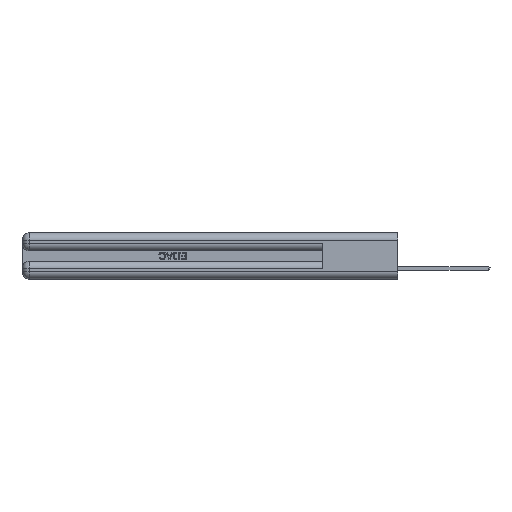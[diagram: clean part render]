
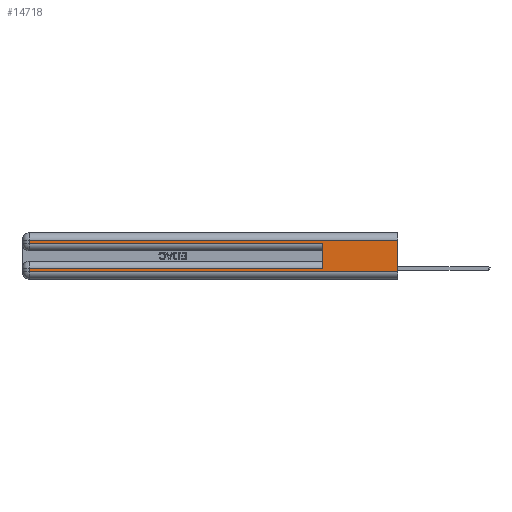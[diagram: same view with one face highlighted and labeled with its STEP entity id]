
A CAD part, left-side view. The second image highlights one B-rep face of the part: STEP entity #14718.
In plain terms, the highlighted planar face has unit normal (-1, 0, 0).
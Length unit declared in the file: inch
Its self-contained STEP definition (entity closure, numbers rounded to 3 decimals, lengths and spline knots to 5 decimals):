
#203 = CARTESIAN_POINT ( 'NONE',  ( 0., 2.94, 0.085 ) ) ;
#742 = DIRECTION ( 'NONE',  ( 0., 0., -1. ) ) ;
#860 = LINE ( 'NONE', #17339, #7563 ) ;
#980 = CARTESIAN_POINT ( 'NONE',  ( 0., 0., 0.06 ) ) ;
#1661 = LINE ( 'NONE', #35250, #13268 ) ;
#1668 = VECTOR ( 'NONE', #10809, 39.37008 ) ;
#3809 = VERTEX_POINT ( 'NONE', #30040 ) ;
#4321 = CARTESIAN_POINT ( 'NONE',  ( 0., 2.94, 0.37 ) ) ;
#5462 = VECTOR ( 'NONE', #8074, 39.37008 ) ;
#6271 = EDGE_CURVE ( 'NONE', #26611, #9084, #42999, .T. ) ;
#6389 = LINE ( 'NONE', #4321, #44031 ) ;
#6460 = CARTESIAN_POINT ( 'NONE',  ( 0., 2.94, 0.31 ) ) ;
#7563 = VECTOR ( 'NONE', #25642, 39.37008 ) ;
#8074 = DIRECTION ( 'NONE',  ( 0., 0., 1. ) ) ;
#8088 = DIRECTION ( 'NONE',  ( 0., 0., -1. ) ) ;
#8125 = FACE_OUTER_BOUND ( 'NONE', #28243, .T. ) ;
#9084 = VERTEX_POINT ( 'NONE', #203 ) ;
#9880 = ORIENTED_EDGE ( 'NONE', *, *, #37653, .T. ) ;
#10809 = DIRECTION ( 'NONE',  ( 0., 1., 0. ) ) ;
#11498 = CARTESIAN_POINT ( 'NONE',  ( 0., 0., 0.285 ) ) ;
#12879 = CARTESIAN_POINT ( 'NONE',  ( 0., 0.6, 0.285 ) ) ;
#13268 = VECTOR ( 'NONE', #23384, 39.37008 ) ;
#13643 = LINE ( 'NONE', #980, #31822 ) ;
#13735 = EDGE_CURVE ( 'NONE', #47105, #3809, #34945, .T. ) ;
#14718 = ADVANCED_FACE ( 'NONE', ( #8125 ), #19404, .F. ) ;
#14836 = VECTOR ( 'NONE', #22846, 39.37008 ) ;
#17339 = CARTESIAN_POINT ( 'NONE',  ( 0., 0., 0.31 ) ) ;
#18374 = EDGE_CURVE ( 'NONE', #9084, #39132, #1661, .T. ) ;
#19404 = PLANE ( 'NONE',  #20004 ) ;
#20004 = AXIS2_PLACEMENT_3D ( 'NONE', #47565, #27796, #742 ) ;
#22846 = DIRECTION ( 'NONE',  ( 0., -1., 0. ) ) ;
#23384 = DIRECTION ( 'NONE',  ( 0., 0., -1. ) ) ;
#23535 = CARTESIAN_POINT ( 'NONE',  ( 0., 0.6, 0.145 ) ) ;
#24640 = VECTOR ( 'NONE', #28387, 39.37008 ) ;
#24663 = ORIENTED_EDGE ( 'NONE', *, *, #18374, .T. ) ;
#25439 = ORIENTED_EDGE ( 'NONE', *, *, #45670, .T. ) ;
#25642 = DIRECTION ( 'NONE',  ( 0., 1., 0. ) ) ;
#26077 = ORIENTED_EDGE ( 'NONE', *, *, #13735, .F. ) ;
#26200 = CARTESIAN_POINT ( 'NONE',  ( 0., 0., 0.085 ) ) ;
#26611 = VERTEX_POINT ( 'NONE', #28772 ) ;
#27796 = DIRECTION ( 'NONE',  ( 1., 0., 0. ) ) ;
#28243 = EDGE_LOOP ( 'NONE', ( #26077, #33607, #42848, #9880, #47006, #39657, #24663, #25439 ) ) ;
#28387 = DIRECTION ( 'NONE',  ( 0., 0., -1. ) ) ;
#28772 = CARTESIAN_POINT ( 'NONE',  ( 0., 0.6, 0.085 ) ) ;
#30040 = CARTESIAN_POINT ( 'NONE',  ( 0., 0., 0.06 ) ) ;
#31822 = VECTOR ( 'NONE', #43453, 39.37008 ) ;
#32595 = VERTEX_POINT ( 'NONE', #43047 ) ;
#33607 = ORIENTED_EDGE ( 'NONE', *, *, #40633, .T. ) ;
#34759 = CARTESIAN_POINT ( 'NONE',  ( 0., 0., 0.31 ) ) ;
#34945 = LINE ( 'NONE', #39729, #24640 ) ;
#35250 = CARTESIAN_POINT ( 'NONE',  ( 0., 2.94, 0.37 ) ) ;
#35533 = VERTEX_POINT ( 'NONE', #12879 ) ;
#37202 = VERTEX_POINT ( 'NONE', #6460 ) ;
#37653 = EDGE_CURVE ( 'NONE', #32595, #35533, #50067, .T. ) ;
#39132 = VERTEX_POINT ( 'NONE', #49721 ) ;
#39638 = EDGE_CURVE ( 'NONE', #26611, #35533, #47406, .T. ) ;
#39657 = ORIENTED_EDGE ( 'NONE', *, *, #6271, .T. ) ;
#39729 = CARTESIAN_POINT ( 'NONE',  ( 0., 0., 0.37 ) ) ;
#40633 = EDGE_CURVE ( 'NONE', #47105, #37202, #860, .T. ) ;
#42848 = ORIENTED_EDGE ( 'NONE', *, *, #49271, .T. ) ;
#42999 = LINE ( 'NONE', #26200, #1668 ) ;
#43047 = CARTESIAN_POINT ( 'NONE',  ( 0., 2.94, 0.285 ) ) ;
#43453 = DIRECTION ( 'NONE',  ( 0., -1., 0. ) ) ;
#44031 = VECTOR ( 'NONE', #8088, 39.37008 ) ;
#45670 = EDGE_CURVE ( 'NONE', #39132, #3809, #13643, .T. ) ;
#47006 = ORIENTED_EDGE ( 'NONE', *, *, #39638, .F. ) ;
#47105 = VERTEX_POINT ( 'NONE', #34759 ) ;
#47406 = LINE ( 'NONE', #23535, #5462 ) ;
#47565 = CARTESIAN_POINT ( 'NONE',  ( 0., 0., 0.37 ) ) ;
#49271 = EDGE_CURVE ( 'NONE', #37202, #32595, #6389, .T. ) ;
#49721 = CARTESIAN_POINT ( 'NONE',  ( 0., 2.94, 0.06 ) ) ;
#50067 = LINE ( 'NONE', #11498, #14836 ) ;
